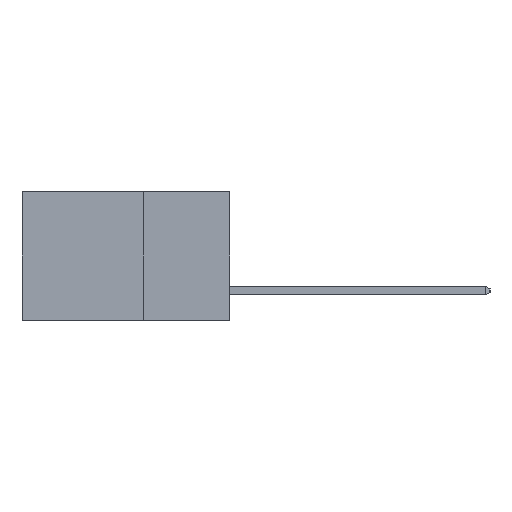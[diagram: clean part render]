
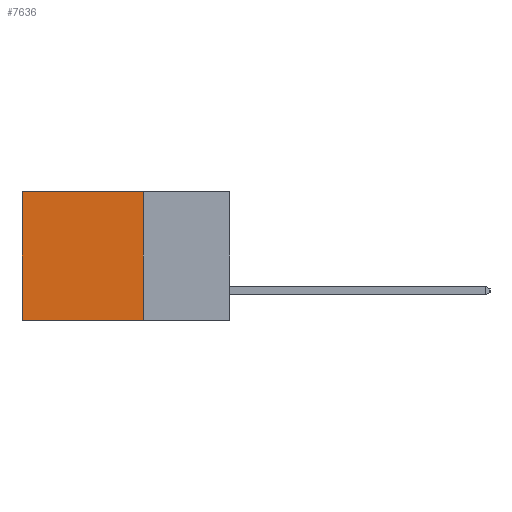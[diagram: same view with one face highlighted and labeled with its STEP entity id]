
A CAD part, left-side view. The second image highlights one B-rep face of the part: STEP entity #7636.
In plain terms, the highlighted planar face has unit normal (-1, 0, 0).
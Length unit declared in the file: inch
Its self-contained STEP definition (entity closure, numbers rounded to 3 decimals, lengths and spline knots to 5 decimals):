
#343 = VERTEX_POINT ( 'NONE', #15509 ) ;
#758 = EDGE_CURVE ( 'NONE', #8412, #6787, #5097, .T. ) ;
#1115 = VECTOR ( 'NONE', #5876, 39.37008 ) ;
#1222 = ORIENTED_EDGE ( 'NONE', *, *, #758, .F. ) ;
#1339 = EDGE_CURVE ( 'NONE', #343, #14610, #10414, .T. ) ;
#2099 = CARTESIAN_POINT ( 'NONE',  ( 0.298, 0.6, 0. ) ) ;
#2292 = VECTOR ( 'NONE', #10516, 39.37008 ) ;
#2416 = CARTESIAN_POINT ( 'NONE',  ( 0.298, 0.25, 0. ) ) ;
#2585 = VECTOR ( 'NONE', #9099, 39.37008 ) ;
#3031 = LINE ( 'NONE', #3338, #2585 ) ;
#3338 = CARTESIAN_POINT ( 'NONE',  ( 0.298, 0.25, -0.37 ) ) ;
#3489 = CARTESIAN_POINT ( 'NONE',  ( 0.298, 0.25, 0. ) ) ;
#5005 = EDGE_CURVE ( 'NONE', #6787, #14610, #3031, .T. ) ;
#5097 = LINE ( 'NONE', #3489, #1115 ) ;
#5876 = DIRECTION ( 'NONE',  ( 0., 0., -1. ) ) ;
#6406 = EDGE_LOOP ( 'NONE', ( #14753, #8921, #1222, #7882 ) ) ;
#6709 = VECTOR ( 'NONE', #17844, 39.37008 ) ;
#6787 = VERTEX_POINT ( 'NONE', #10856 ) ;
#6880 = FACE_OUTER_BOUND ( 'NONE', #6406, .T. ) ;
#7636 = ADVANCED_FACE ( 'NONE', ( #6880 ), #7989, .F. ) ;
#7882 = ORIENTED_EDGE ( 'NONE', *, *, #11863, .T. ) ;
#7989 = PLANE ( 'NONE',  #16662 ) ;
#8412 = VERTEX_POINT ( 'NONE', #2416 ) ;
#8921 = ORIENTED_EDGE ( 'NONE', *, *, #5005, .F. ) ;
#9099 = DIRECTION ( 'NONE',  ( 0., 1., 0. ) ) ;
#9366 = DIRECTION ( 'NONE',  ( 0., 0., -1. ) ) ;
#10414 = LINE ( 'NONE', #2099, #6709 ) ;
#10516 = DIRECTION ( 'NONE',  ( 0., 1., 0. ) ) ;
#10856 = CARTESIAN_POINT ( 'NONE',  ( 0.298, 0.25, -0.37 ) ) ;
#11863 = EDGE_CURVE ( 'NONE', #8412, #343, #17288, .T. ) ;
#14610 = VERTEX_POINT ( 'NONE', #16044 ) ;
#14753 = ORIENTED_EDGE ( 'NONE', *, *, #1339, .T. ) ;
#15509 = CARTESIAN_POINT ( 'NONE',  ( 0.298, 0.6, 0. ) ) ;
#16044 = CARTESIAN_POINT ( 'NONE',  ( 0.298, 0.6, -0.37 ) ) ;
#16051 = CARTESIAN_POINT ( 'NONE',  ( 0.298, 0.25, 0. ) ) ;
#16662 = AXIS2_PLACEMENT_3D ( 'NONE', #17514, #17575, #9366 ) ;
#17288 = LINE ( 'NONE', #16051, #2292 ) ;
#17514 = CARTESIAN_POINT ( 'NONE',  ( 0.298, 0.25, 0. ) ) ;
#17575 = DIRECTION ( 'NONE',  ( 1., 0., 0. ) ) ;
#17844 = DIRECTION ( 'NONE',  ( 0., 0., -1. ) ) ;
